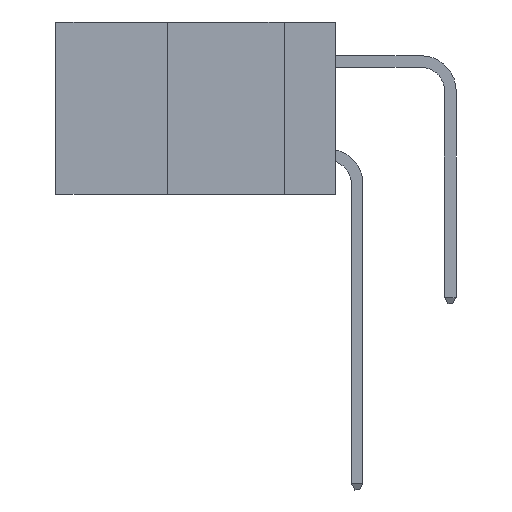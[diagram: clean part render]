
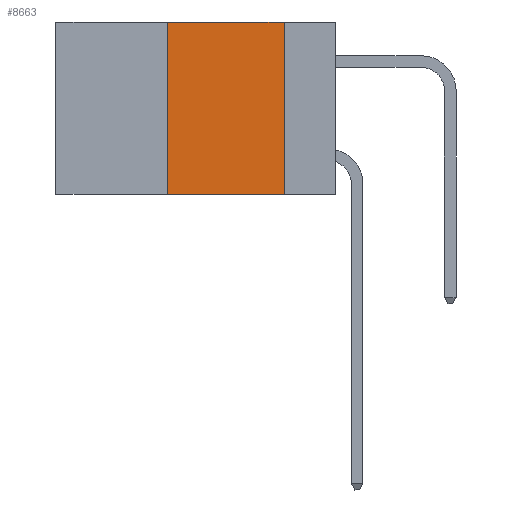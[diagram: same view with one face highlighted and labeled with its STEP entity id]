
A CAD part, left-side view. The second image highlights one B-rep face of the part: STEP entity #8663.
In plain terms, the highlighted planar face has unit normal (-1, 0, 0).
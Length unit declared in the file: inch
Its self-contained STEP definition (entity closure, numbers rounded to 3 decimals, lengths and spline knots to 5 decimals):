
#201 = EDGE_LOOP ( 'NONE', ( #12200, #5643, #17951, #19870 ) ) ;
#321 = PLANE ( 'NONE',  #19620 ) ;
#831 = VECTOR ( 'NONE', #20656, 39.37008 ) ;
#4067 = LINE ( 'NONE', #21742, #8941 ) ;
#4750 = LINE ( 'NONE', #17873, #13508 ) ;
#5027 = DIRECTION ( 'NONE',  ( 1., 0., 0. ) ) ;
#5643 = ORIENTED_EDGE ( 'NONE', *, *, #6805, .F. ) ;
#6805 = EDGE_CURVE ( 'NONE', #11424, #12392, #22568, .T. ) ;
#7365 = CARTESIAN_POINT ( 'NONE',  ( 0., 0.11, 0. ) ) ;
#8445 = VERTEX_POINT ( 'NONE', #22166 ) ;
#8663 = ADVANCED_FACE ( 'NONE', ( #11017 ), #321, .F. ) ;
#8670 = CARTESIAN_POINT ( 'NONE',  ( 0., 0.6, 0. ) ) ;
#8941 = VECTOR ( 'NONE', #13113, 39.37008 ) ;
#9257 = LINE ( 'NONE', #22914, #831 ) ;
#9911 = EDGE_CURVE ( 'NONE', #12392, #8445, #4750, .T. ) ;
#10273 = VERTEX_POINT ( 'NONE', #16928 ) ;
#10749 = EDGE_CURVE ( 'NONE', #10273, #8445, #4067, .T. ) ;
#11017 = FACE_OUTER_BOUND ( 'NONE', #201, .T. ) ;
#11424 = VERTEX_POINT ( 'NONE', #16549 ) ;
#12200 = ORIENTED_EDGE ( 'NONE', *, *, #9911, .F. ) ;
#12392 = VERTEX_POINT ( 'NONE', #7365 ) ;
#13113 = DIRECTION ( 'NONE',  ( 0., -1., 0. ) ) ;
#13508 = VECTOR ( 'NONE', #24178, 39.37008 ) ;
#14845 = DIRECTION ( 'NONE',  ( 0., 0., -1. ) ) ;
#16549 = CARTESIAN_POINT ( 'NONE',  ( 0., 0.36, 0. ) ) ;
#16928 = CARTESIAN_POINT ( 'NONE',  ( 0., 0.36, -0.37 ) ) ;
#17873 = CARTESIAN_POINT ( 'NONE',  ( 0., 0.11, 0. ) ) ;
#17951 = ORIENTED_EDGE ( 'NONE', *, *, #20877, .F. ) ;
#19066 = CARTESIAN_POINT ( 'NONE',  ( 0., 0.6, 0. ) ) ;
#19620 = AXIS2_PLACEMENT_3D ( 'NONE', #8670, #5027, #14845 ) ;
#19870 = ORIENTED_EDGE ( 'NONE', *, *, #10749, .T. ) ;
#20306 = VECTOR ( 'NONE', #21354, 39.37008 ) ;
#20656 = DIRECTION ( 'NONE',  ( 0., 0., 1. ) ) ;
#20877 = EDGE_CURVE ( 'NONE', #10273, #11424, #9257, .T. ) ;
#21354 = DIRECTION ( 'NONE',  ( 0., -1., 0. ) ) ;
#21742 = CARTESIAN_POINT ( 'NONE',  ( 0., 0.6, -0.37 ) ) ;
#22166 = CARTESIAN_POINT ( 'NONE',  ( 0., 0.11, -0.37 ) ) ;
#22568 = LINE ( 'NONE', #19066, #20306 ) ;
#22914 = CARTESIAN_POINT ( 'NONE',  ( 0., 0.36, 0. ) ) ;
#24178 = DIRECTION ( 'NONE',  ( 0., 0., -1. ) ) ;
